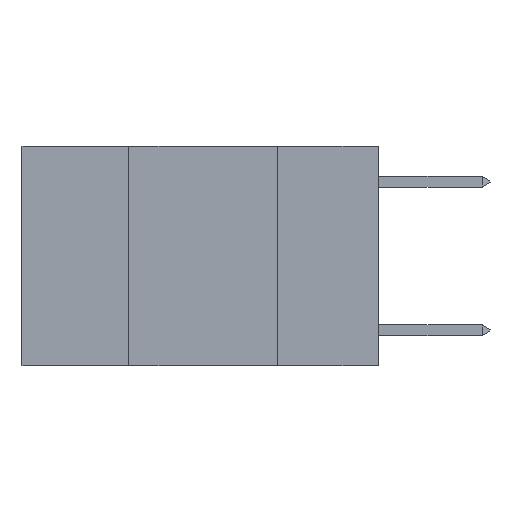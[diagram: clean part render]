
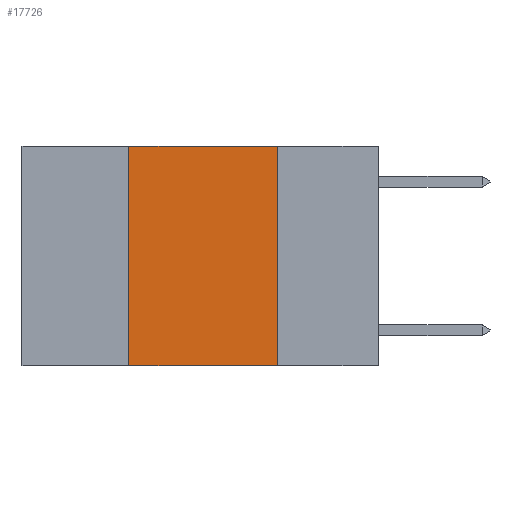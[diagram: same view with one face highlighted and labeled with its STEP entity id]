
A CAD part, left-side view. The second image highlights one B-rep face of the part: STEP entity #17726.
In plain terms, the highlighted planar face has unit normal (-1, 0, 0).
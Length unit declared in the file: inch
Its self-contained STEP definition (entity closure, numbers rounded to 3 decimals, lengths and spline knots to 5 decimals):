
#693 = LINE ( 'NONE', #17649, #2255 ) ;
#875 = CARTESIAN_POINT ( 'NONE',  ( 0., 0.6, -0.37 ) ) ;
#999 = CARTESIAN_POINT ( 'NONE',  ( 0., 0.6, 0. ) ) ;
#1077 = DIRECTION ( 'NONE',  ( 0., -1., 0. ) ) ;
#1232 = ORIENTED_EDGE ( 'NONE', *, *, #8547, .F. ) ;
#1658 = VECTOR ( 'NONE', #12936, 39.37008 ) ;
#2255 = VECTOR ( 'NONE', #10150, 39.37008 ) ;
#2688 = CARTESIAN_POINT ( 'NONE',  ( 0., 0.42, 0. ) ) ;
#2692 = EDGE_CURVE ( 'NONE', #7240, #17021, #19198, .T. ) ;
#3008 = LINE ( 'NONE', #3199, #19267 ) ;
#3199 = CARTESIAN_POINT ( 'NONE',  ( 0., 0.6, 0. ) ) ;
#3656 = CARTESIAN_POINT ( 'NONE',  ( 0., 0.17, 0. ) ) ;
#3658 = ORIENTED_EDGE ( 'NONE', *, *, #12490, .F. ) ;
#4094 = FACE_OUTER_BOUND ( 'NONE', #5336, .T. ) ;
#4540 = ORIENTED_EDGE ( 'NONE', *, *, #6070, .F. ) ;
#5336 = EDGE_LOOP ( 'NONE', ( #1232, #4540, #3658, #12414 ) ) ;
#6070 = EDGE_CURVE ( 'NONE', #7057, #12255, #3008, .T. ) ;
#7038 = CARTESIAN_POINT ( 'NONE',  ( 0., 0.42, -0.37 ) ) ;
#7057 = VERTEX_POINT ( 'NONE', #2688 ) ;
#7240 = VERTEX_POINT ( 'NONE', #7038 ) ;
#8547 = EDGE_CURVE ( 'NONE', #12255, #17021, #11321, .T. ) ;
#10150 = DIRECTION ( 'NONE',  ( 0., 0., 1. ) ) ;
#10797 = CARTESIAN_POINT ( 'NONE',  ( 0., 0.17, -0.37 ) ) ;
#10963 = AXIS2_PLACEMENT_3D ( 'NONE', #999, #11970, #15095 ) ;
#11321 = LINE ( 'NONE', #3656, #1658 ) ;
#11970 = DIRECTION ( 'NONE',  ( 1., 0., 0. ) ) ;
#12255 = VERTEX_POINT ( 'NONE', #15413 ) ;
#12414 = ORIENTED_EDGE ( 'NONE', *, *, #2692, .T. ) ;
#12490 = EDGE_CURVE ( 'NONE', #7240, #7057, #693, .T. ) ;
#12936 = DIRECTION ( 'NONE',  ( 0., 0., -1. ) ) ;
#13281 = PLANE ( 'NONE',  #10963 ) ;
#14834 = DIRECTION ( 'NONE',  ( 0., -1., 0. ) ) ;
#15095 = DIRECTION ( 'NONE',  ( 0., 0., -1. ) ) ;
#15338 = VECTOR ( 'NONE', #1077, 39.37008 ) ;
#15413 = CARTESIAN_POINT ( 'NONE',  ( 0., 0.17, 0. ) ) ;
#17021 = VERTEX_POINT ( 'NONE', #10797 ) ;
#17649 = CARTESIAN_POINT ( 'NONE',  ( 0., 0.42, 0. ) ) ;
#17726 = ADVANCED_FACE ( 'NONE', ( #4094 ), #13281, .F. ) ;
#19198 = LINE ( 'NONE', #875, #15338 ) ;
#19267 = VECTOR ( 'NONE', #14834, 39.37008 ) ;
